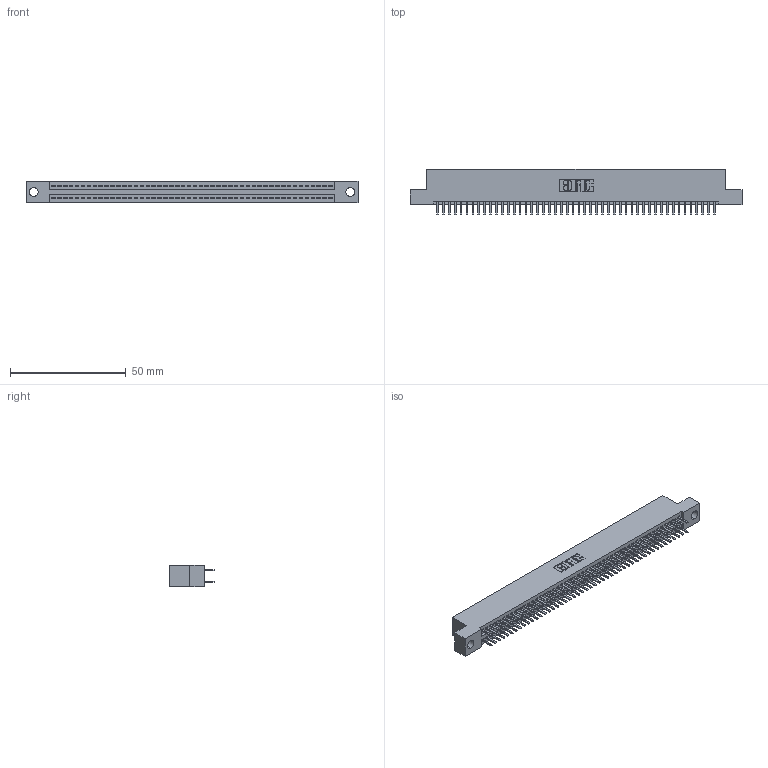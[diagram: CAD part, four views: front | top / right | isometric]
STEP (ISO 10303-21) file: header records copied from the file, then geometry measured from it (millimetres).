
FILE_DESCRIPTION (( 'STEP AP203' ), '1' );
FILE_NAME ('345-096-520-204.STEP', '2021-05-20T16:54:08', ( '' ), ( '' ), 'SwSTEP 2.0', 'SolidWorks 2020', '' );
FILE_SCHEMA (( 'CONFIG_CONTROL_DESIGN' ));
Length unit declared in the file: inch
Products named in the file (3): 345-292-001_345-293-120; 345-096-520-204; 345 Part_Flush Mounting Lugs - 0.156 Dia-TI
Assembly tree (97 placements, depth 2):
  345-096-520-204
    345 Part_Flush Mounting Lugs - 0.156 Dia-TI
    345-292-001_345-293-120  x96
Bounding box: 143.13 x 19.68 x 9.4 mm (x, y, z)
Volume: 13811.2 mm3; surface area: 20293.4 mm2
Topology: 97 solids, 97 shells, 5324 faces, 15449 edges, 10042 vertices
Faces by surface type: plane 3454, cylinder 1870
Entity records: 37387 total; most frequent: CARTESIAN_POINT 6278, ORIENTED_EDGE 6198, DIRECTION 5515, EDGE_CURVE 3099, LINE 2771, VECTOR 2771, VERTEX_POINT 2062, AXIS2_PLACEMENT_3D 1372
